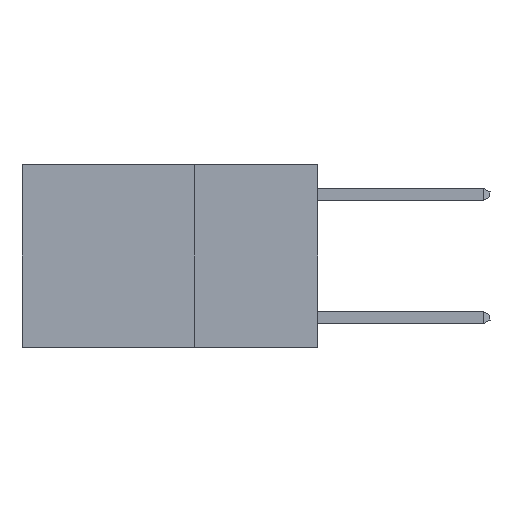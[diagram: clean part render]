
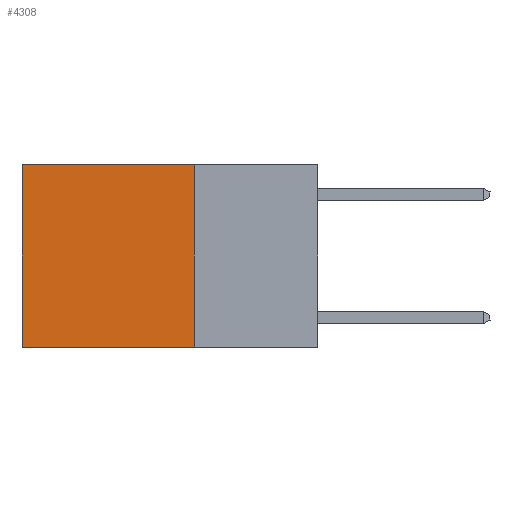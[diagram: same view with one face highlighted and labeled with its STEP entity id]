
A CAD part, left-side view. The second image highlights one B-rep face of the part: STEP entity #4308.
In plain terms, the highlighted planar face has unit normal (-1, 0, 0).
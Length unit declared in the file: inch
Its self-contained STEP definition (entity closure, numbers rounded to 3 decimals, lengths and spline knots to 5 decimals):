
#785 = CARTESIAN_POINT ( 'NONE',  ( 0.2625, 0.25, -0.37 ) ) ;
#971 = CARTESIAN_POINT ( 'NONE',  ( 0.2625, 0.6, 0. ) ) ;
#1728 = CARTESIAN_POINT ( 'NONE',  ( 0.2625, 0.6, 0. ) ) ;
#2148 = CARTESIAN_POINT ( 'NONE',  ( 0.2625, 0.25, 0. ) ) ;
#2149 = LINE ( 'NONE', #14486, #12583 ) ;
#2320 = CARTESIAN_POINT ( 'NONE',  ( 0.2625, 0.25, 0. ) ) ;
#2585 = DIRECTION ( 'NONE',  ( 0., 1., 0. ) ) ;
#2649 = EDGE_CURVE ( 'NONE', #6119, #4164, #7453, .T. ) ;
#3344 = DIRECTION ( 'NONE',  ( 1., 0., 0. ) ) ;
#4164 = VERTEX_POINT ( 'NONE', #14066 ) ;
#4308 = ADVANCED_FACE ( 'NONE', ( #17864 ), #16491, .F. ) ;
#5013 = ORIENTED_EDGE ( 'NONE', *, *, #13699, .T. ) ;
#5063 = CARTESIAN_POINT ( 'NONE',  ( 0.2625, 0.25, 0. ) ) ;
#5132 = LINE ( 'NONE', #2148, #18753 ) ;
#6119 = VERTEX_POINT ( 'NONE', #1728 ) ;
#6830 = DIRECTION ( 'NONE',  ( 0., 0., -1. ) ) ;
#7453 = LINE ( 'NONE', #971, #8573 ) ;
#7597 = CARTESIAN_POINT ( 'NONE',  ( 0.2625, 0.25, 0. ) ) ;
#8109 = ORIENTED_EDGE ( 'NONE', *, *, #19158, .F. ) ;
#8573 = VECTOR ( 'NONE', #20317, 39.37008 ) ;
#10430 = VECTOR ( 'NONE', #2585, 39.37008 ) ;
#10659 = LINE ( 'NONE', #7597, #10430 ) ;
#10938 = EDGE_CURVE ( 'NONE', #13761, #4164, #2149, .T. ) ;
#11939 = AXIS2_PLACEMENT_3D ( 'NONE', #5063, #3344, #14894 ) ;
#12583 = VECTOR ( 'NONE', #18241, 39.37008 ) ;
#13699 = EDGE_CURVE ( 'NONE', #17769, #6119, #10659, .T. ) ;
#13761 = VERTEX_POINT ( 'NONE', #785 ) ;
#14066 = CARTESIAN_POINT ( 'NONE',  ( 0.2625, 0.6, -0.37 ) ) ;
#14486 = CARTESIAN_POINT ( 'NONE',  ( 0.2625, 0.25, -0.37 ) ) ;
#14894 = DIRECTION ( 'NONE',  ( 0., 0., -1. ) ) ;
#16019 = ORIENTED_EDGE ( 'NONE', *, *, #10938, .F. ) ;
#16491 = PLANE ( 'NONE',  #11939 ) ;
#17769 = VERTEX_POINT ( 'NONE', #2320 ) ;
#17864 = FACE_OUTER_BOUND ( 'NONE', #18925, .T. ) ;
#18241 = DIRECTION ( 'NONE',  ( 0., 1., 0. ) ) ;
#18753 = VECTOR ( 'NONE', #6830, 39.37008 ) ;
#18925 = EDGE_LOOP ( 'NONE', ( #20622, #16019, #8109, #5013 ) ) ;
#19158 = EDGE_CURVE ( 'NONE', #17769, #13761, #5132, .T. ) ;
#20317 = DIRECTION ( 'NONE',  ( 0., 0., -1. ) ) ;
#20622 = ORIENTED_EDGE ( 'NONE', *, *, #2649, .T. ) ;
